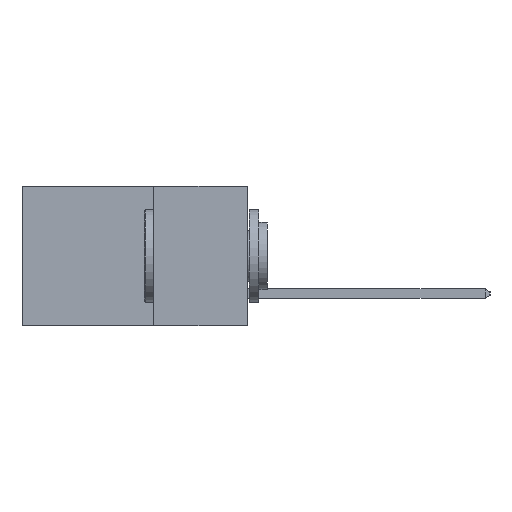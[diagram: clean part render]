
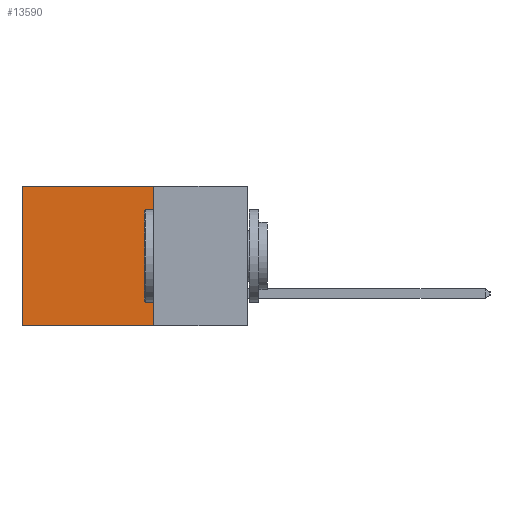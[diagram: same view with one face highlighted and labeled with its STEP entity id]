
A CAD part, left-side view. The second image highlights one B-rep face of the part: STEP entity #13590.
In plain terms, the highlighted planar face has unit normal (-1, 0, 0).
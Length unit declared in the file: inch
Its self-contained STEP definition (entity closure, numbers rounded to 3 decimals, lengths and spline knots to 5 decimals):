
#222 = VERTEX_POINT ( 'NONE', #10993 ) ;
#2497 = DIRECTION ( 'NONE',  ( 0., 0., -1. ) ) ;
#2555 = CARTESIAN_POINT ( 'NONE',  ( 0.2615, 0.25, -0.37 ) ) ;
#2600 = DIRECTION ( 'NONE',  ( 0., 0., -1. ) ) ;
#2646 = CARTESIAN_POINT ( 'NONE',  ( 0.2615, 0.25, 0. ) ) ;
#2889 = CARTESIAN_POINT ( 'NONE',  ( 0.2615, 0.25, -0.37 ) ) ;
#3483 = EDGE_CURVE ( 'NONE', #4998, #222, #17684, .T. ) ;
#3800 = AXIS2_PLACEMENT_3D ( 'NONE', #4468, #4443, #4427 ) ;
#3837 = CARTESIAN_POINT ( 'NONE',  ( 0.2615, 0.6, -0.37 ) ) ;
#4427 = DIRECTION ( 'NONE',  ( 0., 0., -1. ) ) ;
#4435 = FACE_OUTER_BOUND ( 'NONE', #12043, .T. ) ;
#4443 = DIRECTION ( 'NONE',  ( 1., 0., 0. ) ) ;
#4468 = CARTESIAN_POINT ( 'NONE',  ( 0.2615, 0.25, -0.37 ) ) ;
#4743 = PLANE ( 'NONE',  #3800 ) ;
#4977 = VECTOR ( 'NONE', #17832, 39.37008 ) ;
#4998 = VERTEX_POINT ( 'NONE', #2646 ) ;
#5190 = LINE ( 'NONE', #9753, #8119 ) ;
#7136 = VERTEX_POINT ( 'NONE', #3837 ) ;
#7874 = CARTESIAN_POINT ( 'NONE',  ( 0.2615, 0.25, 0. ) ) ;
#8119 = VECTOR ( 'NONE', #2497, 39.37008 ) ;
#8581 = ORIENTED_EDGE ( 'NONE', *, *, #17917, .T. ) ;
#9753 = CARTESIAN_POINT ( 'NONE',  ( 0.2615, 0.6, -0.37 ) ) ;
#9822 = LINE ( 'NONE', #2889, #10280 ) ;
#10280 = VECTOR ( 'NONE', #11659, 39.37008 ) ;
#10993 = CARTESIAN_POINT ( 'NONE',  ( 0.2615, 0.25, -0.37 ) ) ;
#11659 = DIRECTION ( 'NONE',  ( 0., 1., 0. ) ) ;
#12043 = EDGE_LOOP ( 'NONE', ( #13808, #14262, #13856, #8581 ) ) ;
#13590 = ADVANCED_FACE ( 'NONE', ( #4435 ), #4743, .F. ) ;
#13808 = ORIENTED_EDGE ( 'NONE', *, *, #18110, .T. ) ;
#13856 = ORIENTED_EDGE ( 'NONE', *, *, #3483, .F. ) ;
#14262 = ORIENTED_EDGE ( 'NONE', *, *, #17056, .F. ) ;
#15033 = CARTESIAN_POINT ( 'NONE',  ( 0.2615, 0.6, 0. ) ) ;
#16094 = LINE ( 'NONE', #7874, #4977 ) ;
#16153 = VERTEX_POINT ( 'NONE', #15033 ) ;
#17056 = EDGE_CURVE ( 'NONE', #222, #7136, #9822, .T. ) ;
#17284 = VECTOR ( 'NONE', #2600, 39.37008 ) ;
#17684 = LINE ( 'NONE', #2555, #17284 ) ;
#17832 = DIRECTION ( 'NONE',  ( 0., 1., 0. ) ) ;
#17917 = EDGE_CURVE ( 'NONE', #4998, #16153, #16094, .T. ) ;
#18110 = EDGE_CURVE ( 'NONE', #16153, #7136, #5190, .T. ) ;
